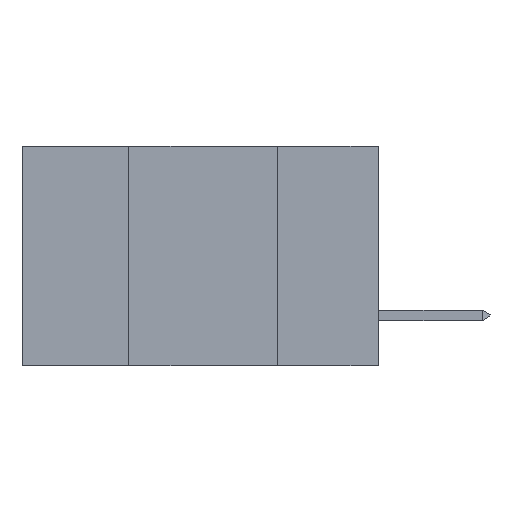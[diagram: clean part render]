
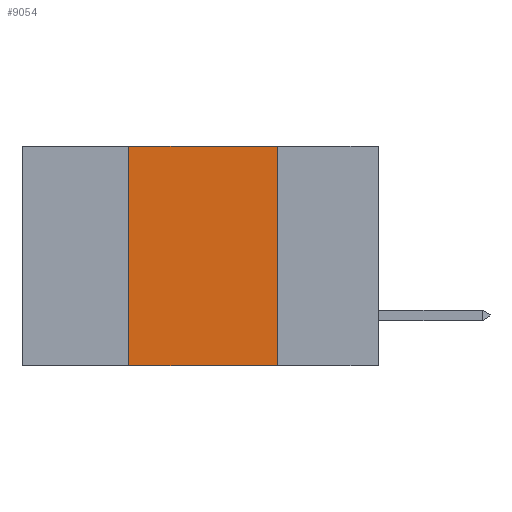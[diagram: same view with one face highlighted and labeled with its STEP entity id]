
A CAD part, left-side view. The second image highlights one B-rep face of the part: STEP entity #9054.
In plain terms, the highlighted planar face has unit normal (-1, 0, 0).
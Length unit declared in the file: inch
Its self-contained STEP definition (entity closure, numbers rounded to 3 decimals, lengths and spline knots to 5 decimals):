
#4317 = LINE ( 'NONE', #9463, #9287 ) ;
#4819 = ORIENTED_EDGE ( 'NONE', *, *, #18566, .F. ) ;
#6191 = EDGE_CURVE ( 'NONE', #11436, #14030, #6512, .T. ) ;
#6512 = LINE ( 'NONE', #13462, #15466 ) ;
#6932 = VERTEX_POINT ( 'NONE', #11072 ) ;
#7469 = DIRECTION ( 'NONE',  ( 0., 0., -1. ) ) ;
#8329 = PLANE ( 'NONE',  #15868 ) ;
#8390 = CARTESIAN_POINT ( 'NONE',  ( 0., 0.6, 0. ) ) ;
#8762 = CARTESIAN_POINT ( 'NONE',  ( 0., 0.42, -0.37 ) ) ;
#8833 = CARTESIAN_POINT ( 'NONE',  ( 0., 0.17, 0. ) ) ;
#9054 = ADVANCED_FACE ( 'NONE', ( #10874 ), #8329, .F. ) ;
#9287 = VECTOR ( 'NONE', #15037, 39.37008 ) ;
#9463 = CARTESIAN_POINT ( 'NONE',  ( 0., 0.6, -0.37 ) ) ;
#9514 = EDGE_CURVE ( 'NONE', #11436, #17173, #4317, .T. ) ;
#9687 = LINE ( 'NONE', #10378, #15291 ) ;
#9782 = DIRECTION ( 'NONE',  ( 0., 0., -1. ) ) ;
#10378 = CARTESIAN_POINT ( 'NONE',  ( 0., 0.6, 0. ) ) ;
#10420 = EDGE_CURVE ( 'NONE', #14030, #6932, #9687, .T. ) ;
#10551 = CARTESIAN_POINT ( 'NONE',  ( 0., 0.17, -0.37 ) ) ;
#10874 = FACE_OUTER_BOUND ( 'NONE', #14578, .T. ) ;
#11072 = CARTESIAN_POINT ( 'NONE',  ( 0., 0.17, 0. ) ) ;
#11093 = ORIENTED_EDGE ( 'NONE', *, *, #6191, .F. ) ;
#11436 = VERTEX_POINT ( 'NONE', #8762 ) ;
#13412 = CARTESIAN_POINT ( 'NONE',  ( 0., 0.42, 0. ) ) ;
#13439 = DIRECTION ( 'NONE',  ( 0., -1., 0. ) ) ;
#13462 = CARTESIAN_POINT ( 'NONE',  ( 0., 0.42, 0. ) ) ;
#14030 = VERTEX_POINT ( 'NONE', #13412 ) ;
#14578 = EDGE_LOOP ( 'NONE', ( #4819, #15116, #11093, #15236 ) ) ;
#15037 = DIRECTION ( 'NONE',  ( 0., -1., 0. ) ) ;
#15116 = ORIENTED_EDGE ( 'NONE', *, *, #10420, .F. ) ;
#15236 = ORIENTED_EDGE ( 'NONE', *, *, #9514, .T. ) ;
#15291 = VECTOR ( 'NONE', #13439, 39.37008 ) ;
#15466 = VECTOR ( 'NONE', #16346, 39.37008 ) ;
#15868 = AXIS2_PLACEMENT_3D ( 'NONE', #8390, #18379, #9782 ) ;
#16346 = DIRECTION ( 'NONE',  ( 0., 0., 1. ) ) ;
#16848 = LINE ( 'NONE', #8833, #17296 ) ;
#17173 = VERTEX_POINT ( 'NONE', #10551 ) ;
#17296 = VECTOR ( 'NONE', #7469, 39.37008 ) ;
#18379 = DIRECTION ( 'NONE',  ( 1., 0., 0. ) ) ;
#18566 = EDGE_CURVE ( 'NONE', #6932, #17173, #16848, .T. ) ;
